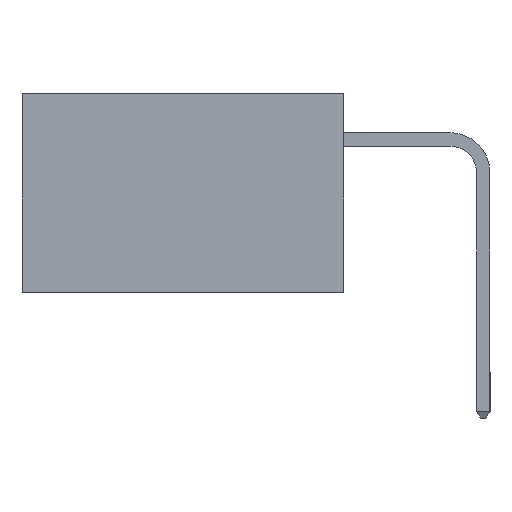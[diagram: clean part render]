
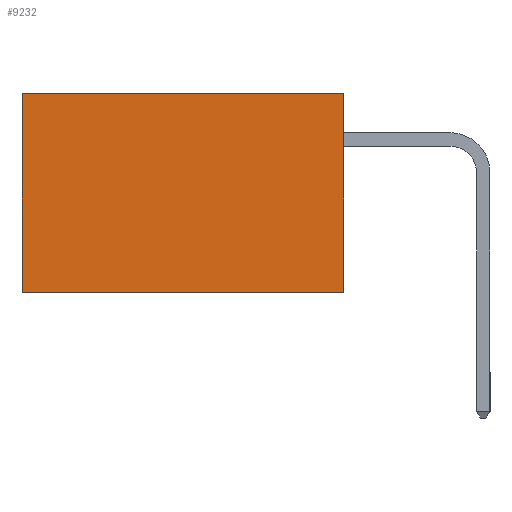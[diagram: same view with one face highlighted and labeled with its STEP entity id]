
A CAD part, left-side view. The second image highlights one B-rep face of the part: STEP entity #9232.
In plain terms, the highlighted planar face has unit normal (-1, 0, 0).
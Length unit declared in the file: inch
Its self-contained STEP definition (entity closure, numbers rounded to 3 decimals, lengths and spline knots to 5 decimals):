
#87 = AXIS2_PLACEMENT_3D ( 'NONE', #10453, #8351, #4043 ) ;
#213 = EDGE_LOOP ( 'NONE', ( #9652, #603, #2616, #1167 ) ) ;
#216 = FACE_OUTER_BOUND ( 'NONE', #213, .T. ) ;
#277 = CARTESIAN_POINT ( 'NONE',  ( 0.2615, 0., -0.37 ) ) ;
#314 = EDGE_CURVE ( 'NONE', #8671, #8147, #6667, .T. ) ;
#603 = ORIENTED_EDGE ( 'NONE', *, *, #4559, .F. ) ;
#636 = VERTEX_POINT ( 'NONE', #8317 ) ;
#1167 = ORIENTED_EDGE ( 'NONE', *, *, #5705, .T. ) ;
#1275 = VECTOR ( 'NONE', #6281, 39.37008 ) ;
#1422 = EDGE_CURVE ( 'NONE', #1909, #636, #3580, .T. ) ;
#1909 = VERTEX_POINT ( 'NONE', #9760 ) ;
#2354 = LINE ( 'NONE', #8416, #5981 ) ;
#2616 = ORIENTED_EDGE ( 'NONE', *, *, #314, .F. ) ;
#2739 = CARTESIAN_POINT ( 'NONE',  ( 0.2615, 0.6, -0.37 ) ) ;
#3580 = LINE ( 'NONE', #2739, #1275 ) ;
#3631 = PLANE ( 'NONE',  #87 ) ;
#4043 = DIRECTION ( 'NONE',  ( 0., 0., -1. ) ) ;
#4559 = EDGE_CURVE ( 'NONE', #8147, #636, #8591, .T. ) ;
#5053 = DIRECTION ( 'NONE',  ( 0., 0., -1. ) ) ;
#5705 = EDGE_CURVE ( 'NONE', #8671, #1909, #2354, .T. ) ;
#5783 = DIRECTION ( 'NONE',  ( 0., 1., 0. ) ) ;
#5981 = VECTOR ( 'NONE', #5783, 39.37008 ) ;
#6281 = DIRECTION ( 'NONE',  ( 0., 0., -1. ) ) ;
#6572 = CARTESIAN_POINT ( 'NONE',  ( 0.2615, 0., -0.37 ) ) ;
#6667 = LINE ( 'NONE', #6572, #7520 ) ;
#7520 = VECTOR ( 'NONE', #5053, 39.37008 ) ;
#7933 = DIRECTION ( 'NONE',  ( 0., 1., 0. ) ) ;
#8147 = VERTEX_POINT ( 'NONE', #8501 ) ;
#8317 = CARTESIAN_POINT ( 'NONE',  ( 0.2615, 0.6, -0.37 ) ) ;
#8351 = DIRECTION ( 'NONE',  ( 1., 0., 0. ) ) ;
#8416 = CARTESIAN_POINT ( 'NONE',  ( 0.2615, 0., 0. ) ) ;
#8501 = CARTESIAN_POINT ( 'NONE',  ( 0.2615, 0., -0.37 ) ) ;
#8591 = LINE ( 'NONE', #277, #9522 ) ;
#8671 = VERTEX_POINT ( 'NONE', #9699 ) ;
#9232 = ADVANCED_FACE ( 'NONE', ( #216 ), #3631, .F. ) ;
#9522 = VECTOR ( 'NONE', #7933, 39.37008 ) ;
#9652 = ORIENTED_EDGE ( 'NONE', *, *, #1422, .T. ) ;
#9699 = CARTESIAN_POINT ( 'NONE',  ( 0.2615, 0., 0. ) ) ;
#9760 = CARTESIAN_POINT ( 'NONE',  ( 0.2615, 0.6, 0. ) ) ;
#10453 = CARTESIAN_POINT ( 'NONE',  ( 0.2615, 0., -0.37 ) ) ;
